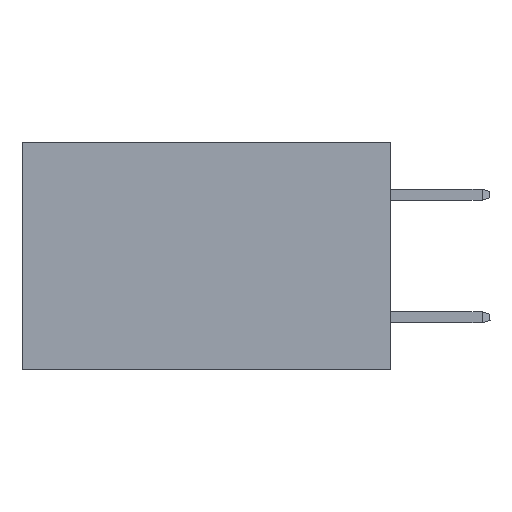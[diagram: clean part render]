
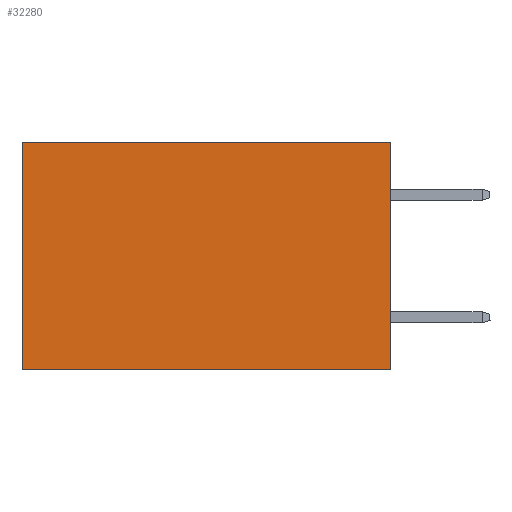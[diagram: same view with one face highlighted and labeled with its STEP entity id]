
A CAD part, left-side view. The second image highlights one B-rep face of the part: STEP entity #32280.
In plain terms, the highlighted planar face has unit normal (-1, 0, 0).
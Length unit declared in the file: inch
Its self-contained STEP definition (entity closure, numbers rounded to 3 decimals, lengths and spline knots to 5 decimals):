
#1355 = EDGE_CURVE ( 'NONE', #15198, #27390, #18935, .T. ) ;
#1652 = LINE ( 'NONE', #10489, #25785 ) ;
#1974 = CARTESIAN_POINT ( 'NONE',  ( 0.2875, 0.6, 0. ) ) ;
#2540 = CARTESIAN_POINT ( 'NONE',  ( 0.2875, 0., -0.37 ) ) ;
#3904 = DIRECTION ( 'NONE',  ( 0., 0., -1. ) ) ;
#4226 = CARTESIAN_POINT ( 'NONE',  ( 0.2875, 0., 0. ) ) ;
#4229 = EDGE_CURVE ( 'NONE', #10802, #16462, #31397, .T. ) ;
#4352 = CARTESIAN_POINT ( 'NONE',  ( 0.2875, 0., 0. ) ) ;
#4766 = VECTOR ( 'NONE', #31582, 39.37008 ) ;
#5064 = DIRECTION ( 'NONE',  ( 0., 1., 0. ) ) ;
#5531 = VECTOR ( 'NONE', #23501, 39.37008 ) ;
#7517 = AXIS2_PLACEMENT_3D ( 'NONE', #4226, #26779, #3904 ) ;
#8103 = CARTESIAN_POINT ( 'NONE',  ( 0.2875, 0.6, -0.37 ) ) ;
#9374 = ORIENTED_EDGE ( 'NONE', *, *, #1355, .T. ) ;
#10489 = CARTESIAN_POINT ( 'NONE',  ( 0.2875, 0., 0. ) ) ;
#10802 = VERTEX_POINT ( 'NONE', #26084 ) ;
#12717 = ORIENTED_EDGE ( 'NONE', *, *, #24329, .F. ) ;
#13501 = CARTESIAN_POINT ( 'NONE',  ( 0.2875, 0., 0. ) ) ;
#13582 = EDGE_LOOP ( 'NONE', ( #24047, #25185, #12717, #9374 ) ) ;
#15198 = VERTEX_POINT ( 'NONE', #4352 ) ;
#15787 = CARTESIAN_POINT ( 'NONE',  ( 0.2875, 0.6, 0. ) ) ;
#16462 = VERTEX_POINT ( 'NONE', #8103 ) ;
#18935 = LINE ( 'NONE', #13501, #4766 ) ;
#21971 = PLANE ( 'NONE',  #7517 ) ;
#22643 = VECTOR ( 'NONE', #5064, 39.37008 ) ;
#23209 = DIRECTION ( 'NONE',  ( 0., 0., -1. ) ) ;
#23501 = DIRECTION ( 'NONE',  ( 0., 0., -1. ) ) ;
#24047 = ORIENTED_EDGE ( 'NONE', *, *, #25660, .T. ) ;
#24329 = EDGE_CURVE ( 'NONE', #15198, #10802, #1652, .T. ) ;
#25086 = FACE_OUTER_BOUND ( 'NONE', #13582, .T. ) ;
#25185 = ORIENTED_EDGE ( 'NONE', *, *, #4229, .F. ) ;
#25660 = EDGE_CURVE ( 'NONE', #27390, #16462, #28111, .T. ) ;
#25785 = VECTOR ( 'NONE', #23209, 39.37008 ) ;
#26084 = CARTESIAN_POINT ( 'NONE',  ( 0.2875, 0., -0.37 ) ) ;
#26779 = DIRECTION ( 'NONE',  ( 1., 0., 0. ) ) ;
#27390 = VERTEX_POINT ( 'NONE', #1974 ) ;
#28111 = LINE ( 'NONE', #15787, #5531 ) ;
#31397 = LINE ( 'NONE', #2540, #22643 ) ;
#31582 = DIRECTION ( 'NONE',  ( 0., 1., 0. ) ) ;
#32280 = ADVANCED_FACE ( 'NONE', ( #25086 ), #21971, .F. ) ;
